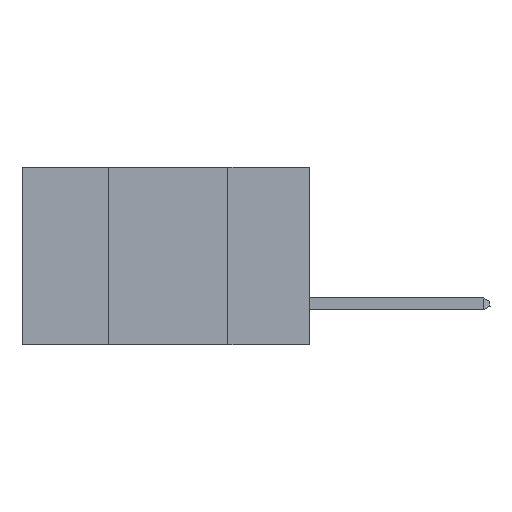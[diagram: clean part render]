
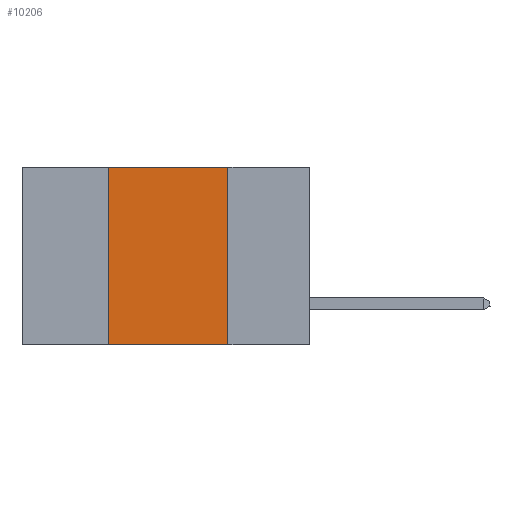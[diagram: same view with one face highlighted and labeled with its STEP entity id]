
A CAD part, left-side view. The second image highlights one B-rep face of the part: STEP entity #10206.
In plain terms, the highlighted planar face has unit normal (-1, 0, 0).
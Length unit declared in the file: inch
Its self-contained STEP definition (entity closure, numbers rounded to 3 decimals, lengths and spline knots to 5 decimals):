
#362 = CARTESIAN_POINT ( 'NONE',  ( 0., 0.6, 0. ) ) ;
#599 = VECTOR ( 'NONE', #9483, 39.37008 ) ;
#760 = LINE ( 'NONE', #3767, #12412 ) ;
#836 = EDGE_CURVE ( 'NONE', #1825, #1156, #6944, .T. ) ;
#861 = FACE_OUTER_BOUND ( 'NONE', #4754, .T. ) ;
#1156 = VERTEX_POINT ( 'NONE', #5715 ) ;
#1288 = EDGE_CURVE ( 'NONE', #10711, #3949, #760, .T. ) ;
#1302 = DIRECTION ( 'NONE',  ( 1., 0., 0. ) ) ;
#1674 = AXIS2_PLACEMENT_3D ( 'NONE', #3542, #1302, #5540 ) ;
#1825 = VERTEX_POINT ( 'NONE', #3703 ) ;
#2294 = EDGE_CURVE ( 'NONE', #3949, #1825, #9924, .T. ) ;
#2432 = DIRECTION ( 'NONE',  ( 0., -1., 0. ) ) ;
#3542 = CARTESIAN_POINT ( 'NONE',  ( 0., 0.6, 0. ) ) ;
#3703 = CARTESIAN_POINT ( 'NONE',  ( 0., 0.17, 0. ) ) ;
#3767 = CARTESIAN_POINT ( 'NONE',  ( 0., 0.42, 0. ) ) ;
#3844 = VECTOR ( 'NONE', #6230, 39.37008 ) ;
#3949 = VERTEX_POINT ( 'NONE', #11212 ) ;
#4754 = EDGE_LOOP ( 'NONE', ( #8520, #11048, #10168, #4873 ) ) ;
#4873 = ORIENTED_EDGE ( 'NONE', *, *, #5878, .T. ) ;
#5540 = DIRECTION ( 'NONE',  ( 0., 0., -1. ) ) ;
#5715 = CARTESIAN_POINT ( 'NONE',  ( 0., 0.17, -0.37 ) ) ;
#5878 = EDGE_CURVE ( 'NONE', #10711, #1156, #6668, .T. ) ;
#6082 = VECTOR ( 'NONE', #2432, 39.37008 ) ;
#6230 = DIRECTION ( 'NONE',  ( 0., -1., 0. ) ) ;
#6668 = LINE ( 'NONE', #12611, #3844 ) ;
#6926 = DIRECTION ( 'NONE',  ( 0., 0., 1. ) ) ;
#6944 = LINE ( 'NONE', #11549, #599 ) ;
#7860 = PLANE ( 'NONE',  #1674 ) ;
#8520 = ORIENTED_EDGE ( 'NONE', *, *, #836, .F. ) ;
#9483 = DIRECTION ( 'NONE',  ( 0., 0., -1. ) ) ;
#9924 = LINE ( 'NONE', #362, #6082 ) ;
#10168 = ORIENTED_EDGE ( 'NONE', *, *, #1288, .F. ) ;
#10206 = ADVANCED_FACE ( 'NONE', ( #861 ), #7860, .F. ) ;
#10488 = CARTESIAN_POINT ( 'NONE',  ( 0., 0.42, -0.37 ) ) ;
#10711 = VERTEX_POINT ( 'NONE', #10488 ) ;
#11048 = ORIENTED_EDGE ( 'NONE', *, *, #2294, .F. ) ;
#11212 = CARTESIAN_POINT ( 'NONE',  ( 0., 0.42, 0. ) ) ;
#11549 = CARTESIAN_POINT ( 'NONE',  ( 0., 0.17, 0. ) ) ;
#12412 = VECTOR ( 'NONE', #6926, 39.37008 ) ;
#12611 = CARTESIAN_POINT ( 'NONE',  ( 0., 0.6, -0.37 ) ) ;
